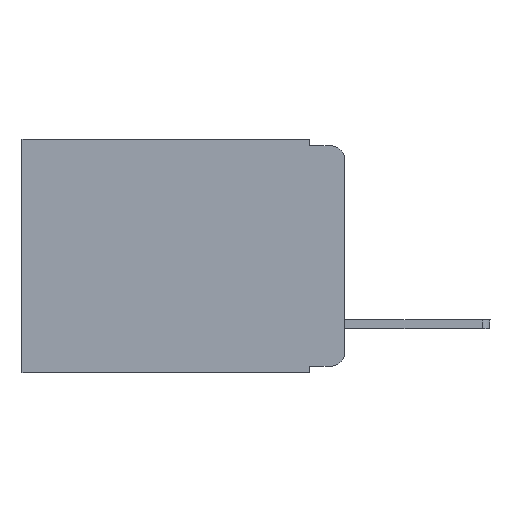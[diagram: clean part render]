
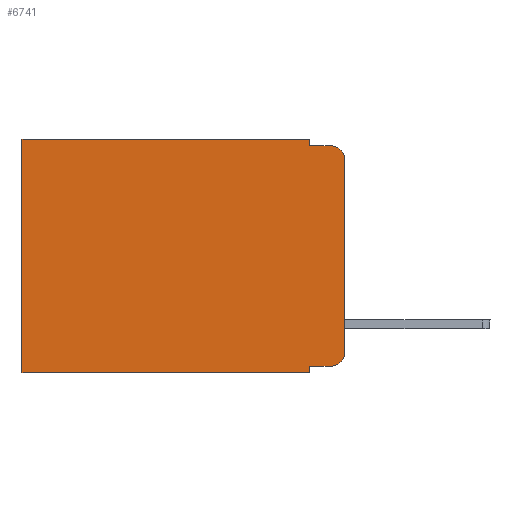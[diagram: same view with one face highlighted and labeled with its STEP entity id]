
A CAD part, left-side view. The second image highlights one B-rep face of the part: STEP entity #6741.
In plain terms, the highlighted planar face has unit normal (-1, 0, 0).
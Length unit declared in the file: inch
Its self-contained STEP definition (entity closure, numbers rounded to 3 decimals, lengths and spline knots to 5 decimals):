
#48 = CARTESIAN_POINT ( 'NONE',  ( 0.298, 0.02, -0.03 ) ) ;
#78 = DIRECTION ( 'NONE',  ( 0., 0., -1. ) ) ;
#598 = LINE ( 'NONE', #10540, #5882 ) ;
#611 = CARTESIAN_POINT ( 'NONE',  ( 0.298, 0.02, -0.313 ) ) ;
#693 = CARTESIAN_POINT ( 'NONE',  ( 0.298, 0.02, -0.01 ) ) ;
#1129 = VECTOR ( 'NONE', #7307, 39.37008 ) ;
#1146 = DIRECTION ( 'NONE',  ( 0., 1., 0. ) ) ;
#1165 = VECTOR ( 'NONE', #2308, 39.37008 ) ;
#1368 = EDGE_CURVE ( 'NONE', #2571, #2843, #3579, .T. ) ;
#1447 = LINE ( 'NONE', #2690, #7655 ) ;
#1492 = EDGE_LOOP ( 'NONE', ( #9640, #5181, #7272, #8291, #6098, #7599, #9265, #10046, #4639, #6638 ) ) ;
#1552 = LINE ( 'NONE', #2223, #1165 ) ;
#1554 = CARTESIAN_POINT ( 'NONE',  ( 0.298, 0.02, -0.333 ) ) ;
#2132 = VERTEX_POINT ( 'NONE', #9809 ) ;
#2142 = CARTESIAN_POINT ( 'NONE',  ( 0.298, 0.051, -0.01 ) ) ;
#2223 = CARTESIAN_POINT ( 'NONE',  ( 0.298, 0.051, -0.333 ) ) ;
#2308 = DIRECTION ( 'NONE',  ( 0., -1., 0. ) ) ;
#2329 = VERTEX_POINT ( 'NONE', #5039 ) ;
#2571 = VERTEX_POINT ( 'NONE', #7850 ) ;
#2690 = CARTESIAN_POINT ( 'NONE',  ( 0.298, 0., 0. ) ) ;
#2801 = VECTOR ( 'NONE', #2860, 39.37008 ) ;
#2843 = VERTEX_POINT ( 'NONE', #3361 ) ;
#2860 = DIRECTION ( 'NONE',  ( 0., -1., 0. ) ) ;
#3086 = EDGE_CURVE ( 'NONE', #7703, #2329, #6989, .T. ) ;
#3146 = PLANE ( 'NONE',  #8244 ) ;
#3361 = CARTESIAN_POINT ( 'NONE',  ( 0.298, 0.473, -0.343 ) ) ;
#3579 = LINE ( 'NONE', #8448, #5548 ) ;
#3664 = CARTESIAN_POINT ( 'NONE',  ( 0.298, 0.051, -0.01 ) ) ;
#3992 = EDGE_CURVE ( 'NONE', #9109, #2843, #4002, .T. ) ;
#4002 = LINE ( 'NONE', #4490, #10371 ) ;
#4008 = CARTESIAN_POINT ( 'NONE',  ( 0.298, 0.051, -0.343 ) ) ;
#4063 = EDGE_CURVE ( 'NONE', #5081, #2571, #6319, .T. ) ;
#4204 = DIRECTION ( 'NONE',  ( 0., 0., -1. ) ) ;
#4247 = EDGE_CURVE ( 'NONE', #7922, #7547, #8517, .T. ) ;
#4490 = CARTESIAN_POINT ( 'NONE',  ( 0.298, 0., -0.343 ) ) ;
#4639 = ORIENTED_EDGE ( 'NONE', *, *, #6747, .T. ) ;
#4697 = VECTOR ( 'NONE', #78, 39.37008 ) ;
#4830 = AXIS2_PLACEMENT_3D ( 'NONE', #611, #4843, #9799 ) ;
#4843 = DIRECTION ( 'NONE',  ( -1., 0., 0. ) ) ;
#4932 = LINE ( 'NONE', #9171, #4697 ) ;
#5039 = CARTESIAN_POINT ( 'NONE',  ( 0.298, 0., -0.313 ) ) ;
#5081 = VERTEX_POINT ( 'NONE', #5832 ) ;
#5181 = ORIENTED_EDGE ( 'NONE', *, *, #5633, .T. ) ;
#5548 = VECTOR ( 'NONE', #6690, 39.37008 ) ;
#5633 = EDGE_CURVE ( 'NONE', #2132, #7547, #8869, .T. ) ;
#5832 = CARTESIAN_POINT ( 'NONE',  ( 0.298, 0.051, 0. ) ) ;
#5853 = DIRECTION ( 'NONE',  ( -1., 0., 0. ) ) ;
#5882 = VECTOR ( 'NONE', #6369, 39.37008 ) ;
#6091 = EDGE_CURVE ( 'NONE', #10050, #9109, #4932, .T. ) ;
#6098 = ORIENTED_EDGE ( 'NONE', *, *, #4063, .T. ) ;
#6150 = EDGE_CURVE ( 'NONE', #2132, #2329, #1447, .T. ) ;
#6319 = LINE ( 'NONE', #10621, #1129 ) ;
#6348 = CARTESIAN_POINT ( 'NONE',  ( 0.298, 0.051, -0.333 ) ) ;
#6369 = DIRECTION ( 'NONE',  ( 0., 0., -1. ) ) ;
#6638 = ORIENTED_EDGE ( 'NONE', *, *, #3086, .T. ) ;
#6690 = DIRECTION ( 'NONE',  ( 0., 0., -1. ) ) ;
#6741 = ADVANCED_FACE ( 'NONE', ( #8961 ), #3146, .F. ) ;
#6747 = EDGE_CURVE ( 'NONE', #10050, #7703, #1552, .T. ) ;
#6989 = CIRCLE ( 'NONE', #4830, 0.02 ) ;
#7272 = ORIENTED_EDGE ( 'NONE', *, *, #4247, .F. ) ;
#7307 = DIRECTION ( 'NONE',  ( 0., 1., 0. ) ) ;
#7320 = DIRECTION ( 'NONE',  ( 1., 0., 0. ) ) ;
#7547 = VERTEX_POINT ( 'NONE', #693 ) ;
#7599 = ORIENTED_EDGE ( 'NONE', *, *, #1368, .T. ) ;
#7626 = DIRECTION ( 'NONE',  ( 0., 0., -1. ) ) ;
#7655 = VECTOR ( 'NONE', #7626, 39.37008 ) ;
#7703 = VERTEX_POINT ( 'NONE', #1554 ) ;
#7850 = CARTESIAN_POINT ( 'NONE',  ( 0.298, 0.473, 0. ) ) ;
#7922 = VERTEX_POINT ( 'NONE', #3664 ) ;
#8149 = DIRECTION ( 'NONE',  ( 0., 0., -1. ) ) ;
#8244 = AXIS2_PLACEMENT_3D ( 'NONE', #8933, #7320, #8149 ) ;
#8291 = ORIENTED_EDGE ( 'NONE', *, *, #9702, .F. ) ;
#8448 = CARTESIAN_POINT ( 'NONE',  ( 0.298, 0.473, 0. ) ) ;
#8517 = LINE ( 'NONE', #2142, #2801 ) ;
#8869 = CIRCLE ( 'NONE', #8902, 0.02 ) ;
#8902 = AXIS2_PLACEMENT_3D ( 'NONE', #48, #5853, #4204 ) ;
#8933 = CARTESIAN_POINT ( 'NONE',  ( 0.298, 0., 0. ) ) ;
#8961 = FACE_OUTER_BOUND ( 'NONE', #1492, .T. ) ;
#9109 = VERTEX_POINT ( 'NONE', #4008 ) ;
#9171 = CARTESIAN_POINT ( 'NONE',  ( 0.298, 0.051, 0. ) ) ;
#9265 = ORIENTED_EDGE ( 'NONE', *, *, #3992, .F. ) ;
#9640 = ORIENTED_EDGE ( 'NONE', *, *, #6150, .F. ) ;
#9702 = EDGE_CURVE ( 'NONE', #5081, #7922, #598, .T. ) ;
#9799 = DIRECTION ( 'NONE',  ( 0., 0., -1. ) ) ;
#9809 = CARTESIAN_POINT ( 'NONE',  ( 0.298, 0., -0.03 ) ) ;
#10046 = ORIENTED_EDGE ( 'NONE', *, *, #6091, .F. ) ;
#10050 = VERTEX_POINT ( 'NONE', #6348 ) ;
#10371 = VECTOR ( 'NONE', #1146, 39.37008 ) ;
#10540 = CARTESIAN_POINT ( 'NONE',  ( 0.298, 0.051, 0. ) ) ;
#10621 = CARTESIAN_POINT ( 'NONE',  ( 0.298, 0., 0. ) ) ;
